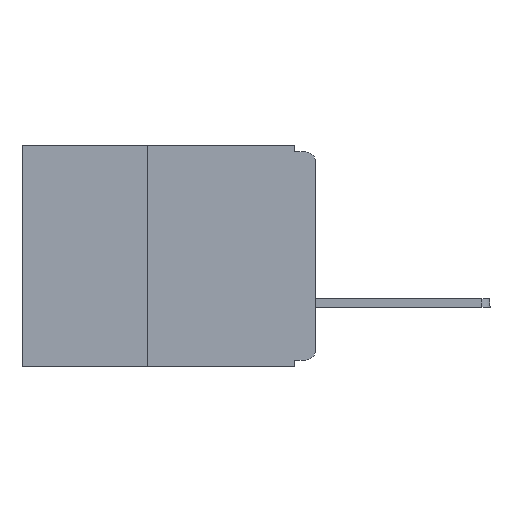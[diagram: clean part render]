
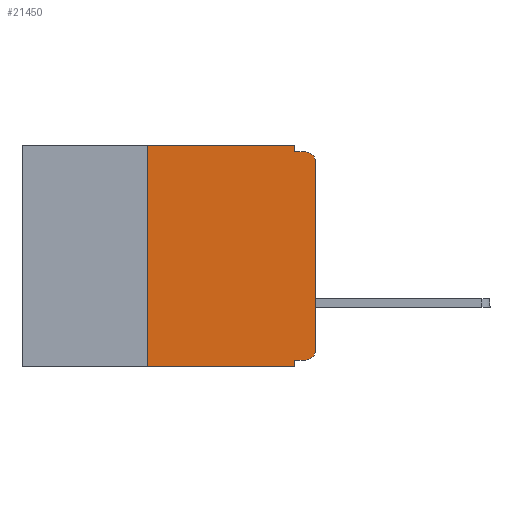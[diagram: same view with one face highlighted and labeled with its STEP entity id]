
A CAD part, left-side view. The second image highlights one B-rep face of the part: STEP entity #21450.
In plain terms, the highlighted planar face has unit normal (-1, 0, 0).
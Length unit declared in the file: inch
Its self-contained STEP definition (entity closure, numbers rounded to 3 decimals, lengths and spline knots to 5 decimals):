
#340 = AXIS2_PLACEMENT_3D ( 'NONE', #15165, #4733, #16871 ) ;
#396 = VERTEX_POINT ( 'NONE', #17038 ) ;
#424 = CARTESIAN_POINT ( 'NONE',  ( 0., 0.031, -0.32 ) ) ;
#891 = VERTEX_POINT ( 'NONE', #16968 ) ;
#1855 = LINE ( 'NONE', #7750, #19274 ) ;
#2054 = CARTESIAN_POINT ( 'NONE',  ( 0., 0.25, -0.33 ) ) ;
#2856 = EDGE_CURVE ( 'NONE', #396, #6060, #13078, .T. ) ;
#3686 = EDGE_CURVE ( 'NONE', #5713, #6060, #19739, .T. ) ;
#4733 = DIRECTION ( 'NONE',  ( -1., 0., 0. ) ) ;
#4961 = ORIENTED_EDGE ( 'NONE', *, *, #8040, .T. ) ;
#5474 = CARTESIAN_POINT ( 'NONE',  ( 0., 0., -0.025 ) ) ;
#5617 = VERTEX_POINT ( 'NONE', #22311 ) ;
#5713 = VERTEX_POINT ( 'NONE', #5474 ) ;
#6027 = ORIENTED_EDGE ( 'NONE', *, *, #3686, .T. ) ;
#6060 = VERTEX_POINT ( 'NONE', #18437 ) ;
#6108 = ORIENTED_EDGE ( 'NONE', *, *, #15688, .F. ) ;
#6200 = VERTEX_POINT ( 'NONE', #20386 ) ;
#6570 = EDGE_CURVE ( 'NONE', #6200, #16545, #1855, .T. ) ;
#6759 = DIRECTION ( 'NONE',  ( 0., 0., -1. ) ) ;
#7076 = CARTESIAN_POINT ( 'NONE',  ( 0., 0., -0.305 ) ) ;
#7123 = LINE ( 'NONE', #9978, #20857 ) ;
#7290 = CARTESIAN_POINT ( 'NONE',  ( 0., 0.031, 0. ) ) ;
#7418 = LINE ( 'NONE', #21280, #20606 ) ;
#7489 = PLANE ( 'NONE',  #16255 ) ;
#7504 = VECTOR ( 'NONE', #10827, 39.37008 ) ;
#7750 = CARTESIAN_POINT ( 'NONE',  ( 0., 0.437, -0.33 ) ) ;
#7761 = VERTEX_POINT ( 'NONE', #424 ) ;
#7768 = VECTOR ( 'NONE', #6759, 39.37008 ) ;
#8035 = ORIENTED_EDGE ( 'NONE', *, *, #10681, .F. ) ;
#8040 = EDGE_CURVE ( 'NONE', #5617, #10774, #21593, .T. ) ;
#8460 = VECTOR ( 'NONE', #10781, 39.37008 ) ;
#8655 = EDGE_LOOP ( 'NONE', ( #13401, #6027, #12000, #12965, #6108, #20630, #11419, #8035, #10288, #4961 ) ) ;
#9205 = FACE_OUTER_BOUND ( 'NONE', #8655, .T. ) ;
#9264 = DIRECTION ( 'NONE',  ( 1., 0., 0. ) ) ;
#9934 = CARTESIAN_POINT ( 'NONE',  ( 0., 0., -0.32 ) ) ;
#9978 = CARTESIAN_POINT ( 'NONE',  ( 0., 0.031, 0. ) ) ;
#10288 = ORIENTED_EDGE ( 'NONE', *, *, #16212, .F. ) ;
#10681 = EDGE_CURVE ( 'NONE', #7761, #16545, #12931, .T. ) ;
#10774 = VERTEX_POINT ( 'NONE', #7076 ) ;
#10781 = DIRECTION ( 'NONE',  ( 0., -1., 0. ) ) ;
#10827 = DIRECTION ( 'NONE',  ( 0., 0., 1. ) ) ;
#11098 = EDGE_CURVE ( 'NONE', #6200, #891, #12121, .T. ) ;
#11154 = LINE ( 'NONE', #9934, #15190 ) ;
#11419 = ORIENTED_EDGE ( 'NONE', *, *, #6570, .T. ) ;
#11615 = AXIS2_PLACEMENT_3D ( 'NONE', #17189, #17182, #17162 ) ;
#11638 = CARTESIAN_POINT ( 'NONE',  ( 0., 0., -0.01 ) ) ;
#11905 = CARTESIAN_POINT ( 'NONE',  ( 0., 0.437, 0. ) ) ;
#12000 = ORIENTED_EDGE ( 'NONE', *, *, #2856, .F. ) ;
#12011 = CARTESIAN_POINT ( 'NONE',  ( 0., 0.031, -0.33 ) ) ;
#12121 = LINE ( 'NONE', #2054, #7504 ) ;
#12931 = LINE ( 'NONE', #12011, #7768 ) ;
#12965 = ORIENTED_EDGE ( 'NONE', *, *, #18965, .F. ) ;
#13078 = LINE ( 'NONE', #11638, #8460 ) ;
#13401 = ORIENTED_EDGE ( 'NONE', *, *, #13604, .T. ) ;
#13485 = VERTEX_POINT ( 'NONE', #7290 ) ;
#13558 = LINE ( 'NONE', #11905, #15181 ) ;
#13604 = EDGE_CURVE ( 'NONE', #10774, #5713, #7418, .T. ) ;
#15165 = CARTESIAN_POINT ( 'NONE',  ( 0., 0.015, -0.305 ) ) ;
#15181 = VECTOR ( 'NONE', #22129, 39.37008 ) ;
#15190 = VECTOR ( 'NONE', #20198, 39.37008 ) ;
#15688 = EDGE_CURVE ( 'NONE', #891, #13485, #13558, .T. ) ;
#16212 = EDGE_CURVE ( 'NONE', #5617, #7761, #11154, .T. ) ;
#16216 = DIRECTION ( 'NONE',  ( 0., 0., 1. ) ) ;
#16255 = AXIS2_PLACEMENT_3D ( 'NONE', #19543, #9264, #21246 ) ;
#16545 = VERTEX_POINT ( 'NONE', #17642 ) ;
#16871 = DIRECTION ( 'NONE',  ( 0., 0., -1. ) ) ;
#16968 = CARTESIAN_POINT ( 'NONE',  ( 0., 0.25, 0. ) ) ;
#17038 = CARTESIAN_POINT ( 'NONE',  ( 0., 0.031, -0.01 ) ) ;
#17162 = DIRECTION ( 'NONE',  ( 0., 0., -1. ) ) ;
#17182 = DIRECTION ( 'NONE',  ( -1., 0., 0. ) ) ;
#17189 = CARTESIAN_POINT ( 'NONE',  ( 0., 0.015, -0.025 ) ) ;
#17642 = CARTESIAN_POINT ( 'NONE',  ( 0., 0.031, -0.33 ) ) ;
#18053 = DIRECTION ( 'NONE',  ( 0., -1., 0. ) ) ;
#18437 = CARTESIAN_POINT ( 'NONE',  ( 0., 0.015, -0.01 ) ) ;
#18520 = DIRECTION ( 'NONE',  ( 0., 0., -1. ) ) ;
#18965 = EDGE_CURVE ( 'NONE', #13485, #396, #7123, .T. ) ;
#19274 = VECTOR ( 'NONE', #18053, 39.37008 ) ;
#19543 = CARTESIAN_POINT ( 'NONE',  ( 0., 0.437, 0. ) ) ;
#19739 = CIRCLE ( 'NONE', #11615, 0.015 ) ;
#20198 = DIRECTION ( 'NONE',  ( 0., 1., 0. ) ) ;
#20386 = CARTESIAN_POINT ( 'NONE',  ( 0., 0.25, -0.33 ) ) ;
#20606 = VECTOR ( 'NONE', #16216, 39.37008 ) ;
#20630 = ORIENTED_EDGE ( 'NONE', *, *, #11098, .F. ) ;
#20857 = VECTOR ( 'NONE', #18520, 39.37008 ) ;
#21246 = DIRECTION ( 'NONE',  ( 0., 0., -1. ) ) ;
#21280 = CARTESIAN_POINT ( 'NONE',  ( 0., 0., 0. ) ) ;
#21450 = ADVANCED_FACE ( 'NONE', ( #9205 ), #7489, .F. ) ;
#21593 = CIRCLE ( 'NONE', #340, 0.015 ) ;
#22129 = DIRECTION ( 'NONE',  ( 0., -1., 0. ) ) ;
#22311 = CARTESIAN_POINT ( 'NONE',  ( 0., 0.015, -0.32 ) ) ;
